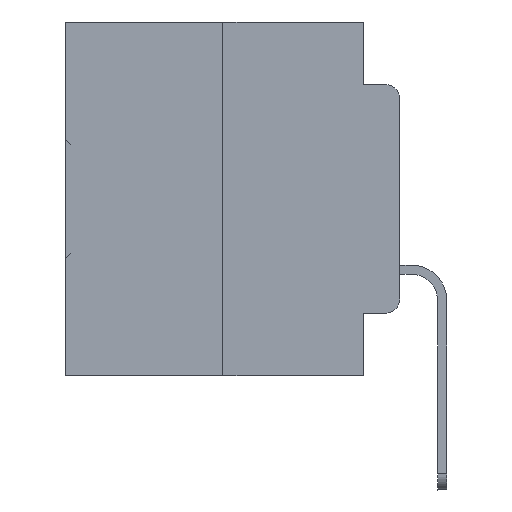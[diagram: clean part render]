
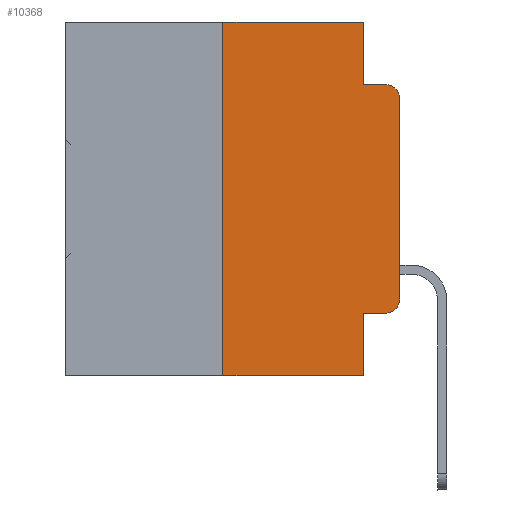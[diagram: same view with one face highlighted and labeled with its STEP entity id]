
A CAD part, left-side view. The second image highlights one B-rep face of the part: STEP entity #10368.
In plain terms, the highlighted planar face has unit normal (-1, 0, 0).
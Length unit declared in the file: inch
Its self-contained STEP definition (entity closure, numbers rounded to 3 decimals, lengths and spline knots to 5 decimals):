
#719 = EDGE_CURVE ( 'NONE', #13626, #32593, #888, .T. ) ;
#850 = VECTOR ( 'NONE', #28557, 39.37008 ) ;
#888 = LINE ( 'NONE', #24019, #2353 ) ;
#1119 = VECTOR ( 'NONE', #15185, 39.37008 ) ;
#1411 = VECTOR ( 'NONE', #4725, 39.37008 ) ;
#1729 = CARTESIAN_POINT ( 'NONE',  ( 0., 0.473, -0.5 ) ) ;
#2001 = VECTOR ( 'NONE', #19774, 39.37008 ) ;
#2353 = VECTOR ( 'NONE', #18435, 39.37008 ) ;
#2737 = LINE ( 'NONE', #23152, #850 ) ;
#2745 = EDGE_LOOP ( 'NONE', ( #28005, #26596, #14989, #23118, #7223, #19840, #27797, #12727, #27524, #12662 ) ) ;
#3076 = DIRECTION ( 'NONE',  ( -1., 0., 0. ) ) ;
#3214 = CARTESIAN_POINT ( 'NONE',  ( 0., 0.473, 0. ) ) ;
#3765 = CIRCLE ( 'NONE', #9212, 0.02 ) ;
#4030 = LINE ( 'NONE', #30538, #1411 ) ;
#4725 = DIRECTION ( 'NONE',  ( 0., 0., 1. ) ) ;
#5128 = CARTESIAN_POINT ( 'NONE',  ( 0., 0.02, -0.3915 ) ) ;
#5493 = CIRCLE ( 'NONE', #22319, 0.02 ) ;
#5965 = CARTESIAN_POINT ( 'NONE',  ( 0., 0.02, -0.1085 ) ) ;
#6277 = EDGE_CURVE ( 'NONE', #8258, #32593, #3765, .T. ) ;
#6354 = DIRECTION ( 'NONE',  ( 0., 0., -1. ) ) ;
#6739 = VECTOR ( 'NONE', #24455, 39.37008 ) ;
#6860 = LINE ( 'NONE', #1729, #27953 ) ;
#7118 = DIRECTION ( 'NONE',  ( 0., 0., -1. ) ) ;
#7142 = VERTEX_POINT ( 'NONE', #13660 ) ;
#7223 = ORIENTED_EDGE ( 'NONE', *, *, #20909, .F. ) ;
#7352 = EDGE_CURVE ( 'NONE', #9390, #8258, #2737, .T. ) ;
#8007 = DIRECTION ( 'NONE',  ( 0., 0., -1. ) ) ;
#8258 = VERTEX_POINT ( 'NONE', #22317 ) ;
#9212 = AXIS2_PLACEMENT_3D ( 'NONE', #5965, #20922, #8007 ) ;
#9388 = CARTESIAN_POINT ( 'NONE',  ( 0., 0.051, -0.0885 ) ) ;
#9390 = VERTEX_POINT ( 'NONE', #20852 ) ;
#10075 = CARTESIAN_POINT ( 'NONE',  ( 0., 0.02, -0.0885 ) ) ;
#10368 = ADVANCED_FACE ( 'NONE', ( #27993 ), #25790, .F. ) ;
#10687 = VERTEX_POINT ( 'NONE', #24577 ) ;
#11106 = LINE ( 'NONE', #11788, #29328 ) ;
#11630 = CARTESIAN_POINT ( 'NONE',  ( 0., 0.25, 0. ) ) ;
#11788 = CARTESIAN_POINT ( 'NONE',  ( 0., 0.051, 0. ) ) ;
#12118 = LINE ( 'NONE', #14506, #1119 ) ;
#12662 = ORIENTED_EDGE ( 'NONE', *, *, #13846, .T. ) ;
#12727 = ORIENTED_EDGE ( 'NONE', *, *, #13623, .F. ) ;
#13538 = EDGE_CURVE ( 'NONE', #20039, #13626, #11106, .T. ) ;
#13623 = EDGE_CURVE ( 'NONE', #32942, #7142, #12118, .T. ) ;
#13626 = VERTEX_POINT ( 'NONE', #9388 ) ;
#13660 = CARTESIAN_POINT ( 'NONE',  ( 0., 0.051, -0.5 ) ) ;
#13846 = EDGE_CURVE ( 'NONE', #28911, #9390, #5493, .T. ) ;
#14506 = CARTESIAN_POINT ( 'NONE',  ( 0., 0.051, 0. ) ) ;
#14989 = ORIENTED_EDGE ( 'NONE', *, *, #719, .F. ) ;
#15009 = EDGE_CURVE ( 'NONE', #10687, #7142, #6860, .T. ) ;
#15185 = DIRECTION ( 'NONE',  ( 0., 0., -1. ) ) ;
#15781 = EDGE_CURVE ( 'NONE', #10687, #19435, #4030, .T. ) ;
#16651 = LINE ( 'NONE', #3214, #6739 ) ;
#16908 = LINE ( 'NONE', #30465, #2001 ) ;
#18285 = EDGE_CURVE ( 'NONE', #32942, #28911, #16908, .T. ) ;
#18435 = DIRECTION ( 'NONE',  ( 0., -1., 0. ) ) ;
#19435 = VERTEX_POINT ( 'NONE', #11630 ) ;
#19774 = DIRECTION ( 'NONE',  ( 0., -1., 0. ) ) ;
#19840 = ORIENTED_EDGE ( 'NONE', *, *, #15781, .F. ) ;
#20032 = CARTESIAN_POINT ( 'NONE',  ( 0., 0.473, 0. ) ) ;
#20039 = VERTEX_POINT ( 'NONE', #30265 ) ;
#20369 = DIRECTION ( 'NONE',  ( 1., 0., 0. ) ) ;
#20852 = CARTESIAN_POINT ( 'NONE',  ( 0., 0., -0.3915 ) ) ;
#20909 = EDGE_CURVE ( 'NONE', #19435, #20039, #16651, .T. ) ;
#20922 = DIRECTION ( 'NONE',  ( -1., 0., 0. ) ) ;
#22317 = CARTESIAN_POINT ( 'NONE',  ( 0., 0., -0.1085 ) ) ;
#22319 = AXIS2_PLACEMENT_3D ( 'NONE', #5128, #3076, #23477 ) ;
#23118 = ORIENTED_EDGE ( 'NONE', *, *, #13538, .F. ) ;
#23152 = CARTESIAN_POINT ( 'NONE',  ( 0., 0., 0. ) ) ;
#23477 = DIRECTION ( 'NONE',  ( 0., 0., -1. ) ) ;
#24019 = CARTESIAN_POINT ( 'NONE',  ( 0., 0.051, -0.0885 ) ) ;
#24455 = DIRECTION ( 'NONE',  ( 0., -1., 0. ) ) ;
#24577 = CARTESIAN_POINT ( 'NONE',  ( 0., 0.25, -0.5 ) ) ;
#25790 = PLANE ( 'NONE',  #27073 ) ;
#26596 = ORIENTED_EDGE ( 'NONE', *, *, #6277, .T. ) ;
#27073 = AXIS2_PLACEMENT_3D ( 'NONE', #20032, #20369, #7118 ) ;
#27524 = ORIENTED_EDGE ( 'NONE', *, *, #18285, .T. ) ;
#27797 = ORIENTED_EDGE ( 'NONE', *, *, #15009, .T. ) ;
#27953 = VECTOR ( 'NONE', #29068, 39.37008 ) ;
#27993 = FACE_OUTER_BOUND ( 'NONE', #2745, .T. ) ;
#28005 = ORIENTED_EDGE ( 'NONE', *, *, #7352, .T. ) ;
#28557 = DIRECTION ( 'NONE',  ( 0., 0., 1. ) ) ;
#28911 = VERTEX_POINT ( 'NONE', #33502 ) ;
#29068 = DIRECTION ( 'NONE',  ( 0., -1., 0. ) ) ;
#29328 = VECTOR ( 'NONE', #6354, 39.37008 ) ;
#30265 = CARTESIAN_POINT ( 'NONE',  ( 0., 0.051, 0. ) ) ;
#30465 = CARTESIAN_POINT ( 'NONE',  ( 0., 0.051, -0.4115 ) ) ;
#30538 = CARTESIAN_POINT ( 'NONE',  ( 0., 0.25, 0. ) ) ;
#32285 = CARTESIAN_POINT ( 'NONE',  ( 0., 0.051, -0.4115 ) ) ;
#32593 = VERTEX_POINT ( 'NONE', #10075 ) ;
#32942 = VERTEX_POINT ( 'NONE', #32285 ) ;
#33502 = CARTESIAN_POINT ( 'NONE',  ( 0., 0.02, -0.4115 ) ) ;
